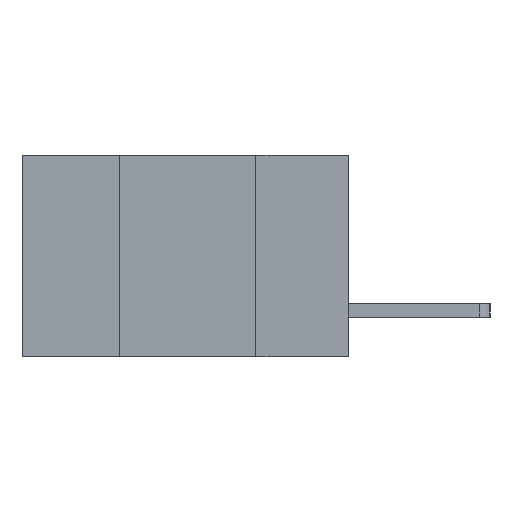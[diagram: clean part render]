
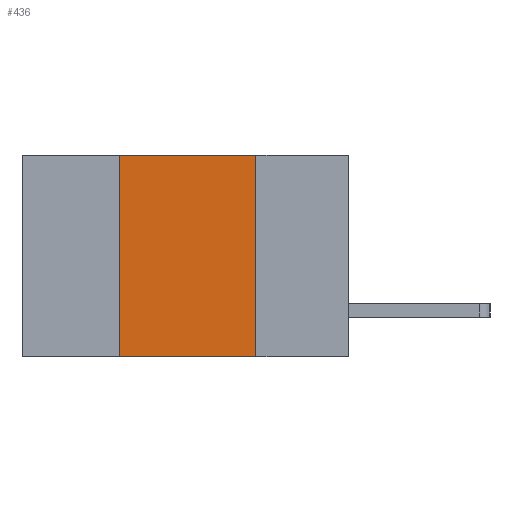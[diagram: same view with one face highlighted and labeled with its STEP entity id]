
A CAD part, left-side view. The second image highlights one B-rep face of the part: STEP entity #436.
In plain terms, the highlighted planar face has unit normal (-1, 0, 0).
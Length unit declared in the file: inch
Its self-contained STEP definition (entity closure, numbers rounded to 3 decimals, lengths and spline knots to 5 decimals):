
#307 = EDGE_CURVE ( 'NONE', #6551, #8067, #7641, .T. ) ;
#436 = ADVANCED_FACE ( 'NONE', ( #4499 ), #8351, .F. ) ;
#1119 = VECTOR ( 'NONE', #6994, 39.37008 ) ;
#3461 = EDGE_LOOP ( 'NONE', ( #8968, #8732, #4507, #6705 ) ) ;
#3962 = VECTOR ( 'NONE', #5737, 39.37008 ) ;
#4069 = CARTESIAN_POINT ( 'NONE',  ( 0., 0.6, -0.37 ) ) ;
#4233 = CARTESIAN_POINT ( 'NONE',  ( 0., 0.17, 0. ) ) ;
#4309 = VECTOR ( 'NONE', #6241, 39.37008 ) ;
#4499 = FACE_OUTER_BOUND ( 'NONE', #3461, .T. ) ;
#4507 = ORIENTED_EDGE ( 'NONE', *, *, #8511, .F. ) ;
#4554 = VERTEX_POINT ( 'NONE', #5049 ) ;
#4976 = CARTESIAN_POINT ( 'NONE',  ( 0., 0.17, -0.37 ) ) ;
#5049 = CARTESIAN_POINT ( 'NONE',  ( 0., 0.42, 0. ) ) ;
#5362 = CARTESIAN_POINT ( 'NONE',  ( 0., 0.42, 0. ) ) ;
#5727 = VERTEX_POINT ( 'NONE', #6144 ) ;
#5737 = DIRECTION ( 'NONE',  ( 0., -1., 0. ) ) ;
#6005 = EDGE_CURVE ( 'NONE', #5727, #8067, #8524, .T. ) ;
#6144 = CARTESIAN_POINT ( 'NONE',  ( 0., 0.42, -0.37 ) ) ;
#6241 = DIRECTION ( 'NONE',  ( 0., 0., 1. ) ) ;
#6483 = VECTOR ( 'NONE', #7468, 39.37008 ) ;
#6551 = VERTEX_POINT ( 'NONE', #4233 ) ;
#6705 = ORIENTED_EDGE ( 'NONE', *, *, #6005, .T. ) ;
#6835 = CARTESIAN_POINT ( 'NONE',  ( 0., 0.17, 0. ) ) ;
#6994 = DIRECTION ( 'NONE',  ( 0., 0., -1. ) ) ;
#7105 = AXIS2_PLACEMENT_3D ( 'NONE', #8593, #8620, #7666 ) ;
#7468 = DIRECTION ( 'NONE',  ( 0., -1., 0. ) ) ;
#7500 = CARTESIAN_POINT ( 'NONE',  ( 0., 0.6, 0. ) ) ;
#7595 = EDGE_CURVE ( 'NONE', #4554, #6551, #8373, .T. ) ;
#7641 = LINE ( 'NONE', #6835, #1119 ) ;
#7666 = DIRECTION ( 'NONE',  ( 0., 0., -1. ) ) ;
#8067 = VERTEX_POINT ( 'NONE', #4976 ) ;
#8351 = PLANE ( 'NONE',  #7105 ) ;
#8373 = LINE ( 'NONE', #7500, #6483 ) ;
#8511 = EDGE_CURVE ( 'NONE', #5727, #4554, #8604, .T. ) ;
#8524 = LINE ( 'NONE', #4069, #3962 ) ;
#8593 = CARTESIAN_POINT ( 'NONE',  ( 0., 0.6, 0. ) ) ;
#8604 = LINE ( 'NONE', #5362, #4309 ) ;
#8620 = DIRECTION ( 'NONE',  ( 1., 0., 0. ) ) ;
#8732 = ORIENTED_EDGE ( 'NONE', *, *, #7595, .F. ) ;
#8968 = ORIENTED_EDGE ( 'NONE', *, *, #307, .F. ) ;
